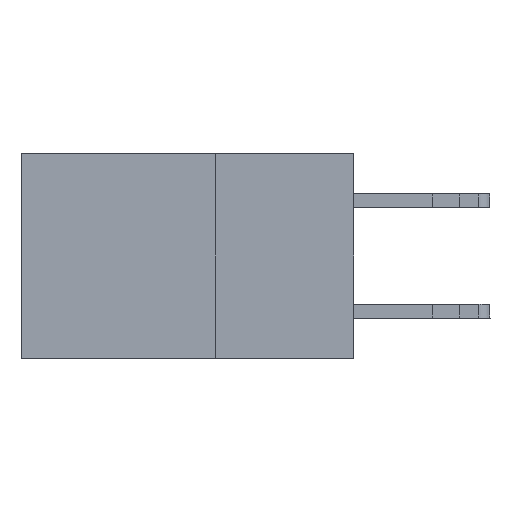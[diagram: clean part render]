
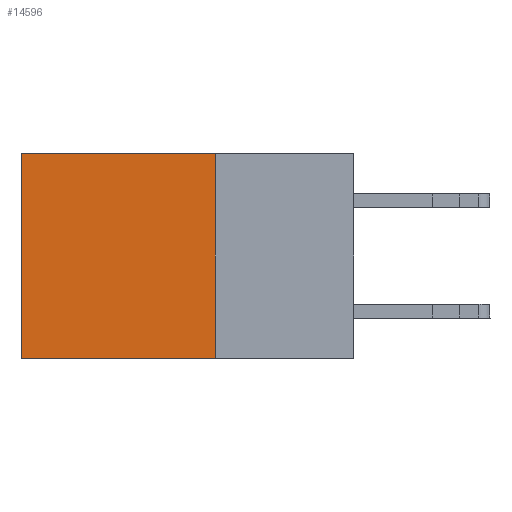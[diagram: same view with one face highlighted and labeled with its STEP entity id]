
A CAD part, left-side view. The second image highlights one B-rep face of the part: STEP entity #14596.
In plain terms, the highlighted planar face has unit normal (-1, 0, 0).
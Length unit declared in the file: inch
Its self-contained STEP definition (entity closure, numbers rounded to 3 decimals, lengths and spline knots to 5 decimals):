
#1152 = DIRECTION ( 'NONE',  ( 0., 1., 0. ) ) ;
#1792 = EDGE_CURVE ( 'NONE', #5370, #19910, #16791, .T. ) ;
#1815 = VERTEX_POINT ( 'NONE', #15273 ) ;
#1827 = ORIENTED_EDGE ( 'NONE', *, *, #8093, .F. ) ;
#3036 = CARTESIAN_POINT ( 'NONE',  ( 0.2875, 0.25, -0.37 ) ) ;
#3961 = ORIENTED_EDGE ( 'NONE', *, *, #8480, .T. ) ;
#4805 = AXIS2_PLACEMENT_3D ( 'NONE', #27010, #22611, #24993 ) ;
#5146 = VECTOR ( 'NONE', #1152, 39.37008 ) ;
#5370 = VERTEX_POINT ( 'NONE', #22170 ) ;
#5713 = CARTESIAN_POINT ( 'NONE',  ( 0.2875, 0.25, -0.37 ) ) ;
#6170 = VECTOR ( 'NONE', #27786, 39.37008 ) ;
#6206 = PLANE ( 'NONE',  #4805 ) ;
#7546 = CARTESIAN_POINT ( 'NONE',  ( 0.2875, 0.25, 0. ) ) ;
#8093 = EDGE_CURVE ( 'NONE', #28482, #19910, #15487, .T. ) ;
#8480 = EDGE_CURVE ( 'NONE', #1815, #5370, #24241, .T. ) ;
#10063 = EDGE_CURVE ( 'NONE', #1815, #28482, #21203, .T. ) ;
#14596 = ADVANCED_FACE ( 'NONE', ( #23396 ), #6206, .F. ) ;
#15273 = CARTESIAN_POINT ( 'NONE',  ( 0.2875, 0.25, 0. ) ) ;
#15487 = LINE ( 'NONE', #5713, #5146 ) ;
#16409 = VECTOR ( 'NONE', #29274, 39.37008 ) ;
#16791 = LINE ( 'NONE', #20050, #16409 ) ;
#16952 = EDGE_LOOP ( 'NONE', ( #17654, #1827, #19106, #3961 ) ) ;
#17654 = ORIENTED_EDGE ( 'NONE', *, *, #1792, .T. ) ;
#19106 = ORIENTED_EDGE ( 'NONE', *, *, #10063, .F. ) ;
#19910 = VERTEX_POINT ( 'NONE', #28518 ) ;
#20050 = CARTESIAN_POINT ( 'NONE',  ( 0.2875, 0.6, 0. ) ) ;
#21203 = LINE ( 'NONE', #27075, #6170 ) ;
#22170 = CARTESIAN_POINT ( 'NONE',  ( 0.2875, 0.6, 0. ) ) ;
#22611 = DIRECTION ( 'NONE',  ( 1., 0., 0. ) ) ;
#23396 = FACE_OUTER_BOUND ( 'NONE', #16952, .T. ) ;
#23939 = DIRECTION ( 'NONE',  ( 0., 1., 0. ) ) ;
#24241 = LINE ( 'NONE', #7546, #27888 ) ;
#24993 = DIRECTION ( 'NONE',  ( 0., 0., -1. ) ) ;
#27010 = CARTESIAN_POINT ( 'NONE',  ( 0.2875, 0.25, 0. ) ) ;
#27075 = CARTESIAN_POINT ( 'NONE',  ( 0.2875, 0.25, 0. ) ) ;
#27786 = DIRECTION ( 'NONE',  ( 0., 0., -1. ) ) ;
#27888 = VECTOR ( 'NONE', #23939, 39.37008 ) ;
#28482 = VERTEX_POINT ( 'NONE', #3036 ) ;
#28518 = CARTESIAN_POINT ( 'NONE',  ( 0.2875, 0.6, -0.37 ) ) ;
#29274 = DIRECTION ( 'NONE',  ( 0., 0., -1. ) ) ;
